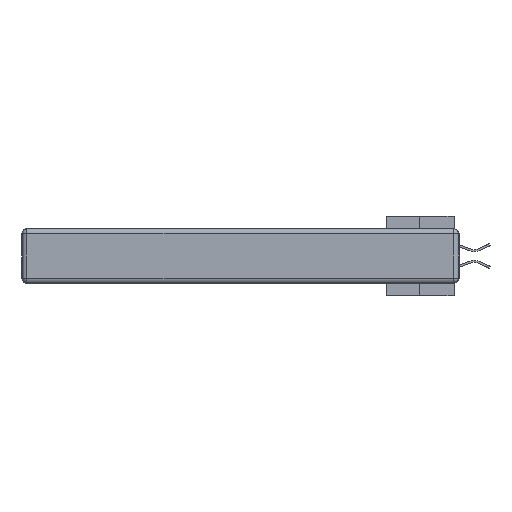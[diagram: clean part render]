
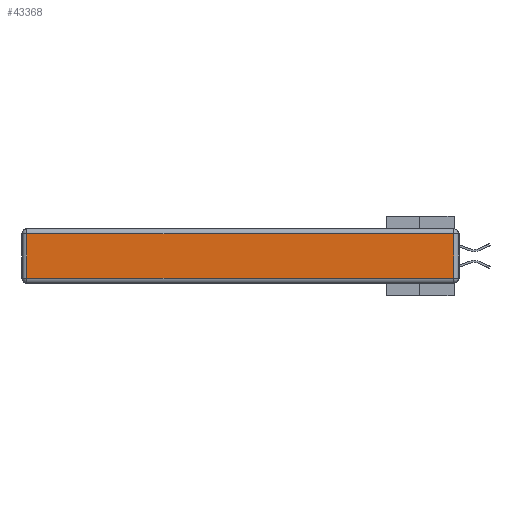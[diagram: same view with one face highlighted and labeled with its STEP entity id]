
A CAD part, left-side view. The second image highlights one B-rep face of the part: STEP entity #43368.
In plain terms, the highlighted planar face has unit normal (-1, 0, 0).
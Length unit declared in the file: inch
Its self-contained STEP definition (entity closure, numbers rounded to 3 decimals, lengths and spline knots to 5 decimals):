
#1085 = CARTESIAN_POINT ( 'NONE',  ( 0., 2.72, -0.03 ) ) ;
#2761 = EDGE_CURVE ( 'NONE', #21145, #4537, #18334, .T. ) ;
#3445 = CARTESIAN_POINT ( 'NONE',  ( 0., 2.72, -0.343 ) ) ;
#4537 = VERTEX_POINT ( 'NONE', #16090 ) ;
#4649 = VECTOR ( 'NONE', #13001, 39.37008 ) ;
#8358 = DIRECTION ( 'NONE',  ( -1., 0., 0. ) ) ;
#8514 = CARTESIAN_POINT ( 'NONE',  ( 0., 2.72, -0.313 ) ) ;
#11394 = ORIENTED_EDGE ( 'NONE', *, *, #27191, .T. ) ;
#13001 = DIRECTION ( 'NONE',  ( 0., 0., 1. ) ) ;
#14932 = VECTOR ( 'NONE', #27277, 39.37008 ) ;
#16090 = CARTESIAN_POINT ( 'NONE',  ( 0., 0.03, -0.03 ) ) ;
#16373 = CARTESIAN_POINT ( 'NONE',  ( 0., 0.03, -0.343 ) ) ;
#17306 = VERTEX_POINT ( 'NONE', #1085 ) ;
#17738 = ORIENTED_EDGE ( 'NONE', *, *, #2761, .T. ) ;
#18101 = LINE ( 'NONE', #3445, #33026 ) ;
#18334 = LINE ( 'NONE', #16373, #4649 ) ;
#19526 = PLANE ( 'NONE',  #24973 ) ;
#21145 = VERTEX_POINT ( 'NONE', #44132 ) ;
#22941 = DIRECTION ( 'NONE',  ( 0., 0., 1. ) ) ;
#24973 = AXIS2_PLACEMENT_3D ( 'NONE', #37534, #8358, #22941 ) ;
#25234 = FACE_OUTER_BOUND ( 'NONE', #28355, .T. ) ;
#27191 = EDGE_CURVE ( 'NONE', #4537, #17306, #44056, .T. ) ;
#27277 = DIRECTION ( 'NONE',  ( 0., -1., 0. ) ) ;
#28355 = EDGE_LOOP ( 'NONE', ( #28927, #17738, #11394, #44382 ) ) ;
#28927 = ORIENTED_EDGE ( 'NONE', *, *, #29248, .T. ) ;
#29248 = EDGE_CURVE ( 'NONE', #44547, #21145, #40792, .T. ) ;
#33026 = VECTOR ( 'NONE', #36285, 39.37008 ) ;
#34524 = CARTESIAN_POINT ( 'NONE',  ( 0., 0., -0.313 ) ) ;
#36285 = DIRECTION ( 'NONE',  ( 0., 0., -1. ) ) ;
#37534 = CARTESIAN_POINT ( 'NONE',  ( 0., 0., -0.343 ) ) ;
#37914 = CARTESIAN_POINT ( 'NONE',  ( 0., 2.75, -0.03 ) ) ;
#39686 = EDGE_CURVE ( 'NONE', #17306, #44547, #18101, .T. ) ;
#40792 = LINE ( 'NONE', #34524, #14932 ) ;
#43368 = ADVANCED_FACE ( 'NONE', ( #25234 ), #19526, .T. ) ;
#43478 = VECTOR ( 'NONE', #45623, 39.37008 ) ;
#44056 = LINE ( 'NONE', #37914, #43478 ) ;
#44132 = CARTESIAN_POINT ( 'NONE',  ( 0., 0.03, -0.313 ) ) ;
#44382 = ORIENTED_EDGE ( 'NONE', *, *, #39686, .T. ) ;
#44547 = VERTEX_POINT ( 'NONE', #8514 ) ;
#45623 = DIRECTION ( 'NONE',  ( 0., 1., 0. ) ) ;
